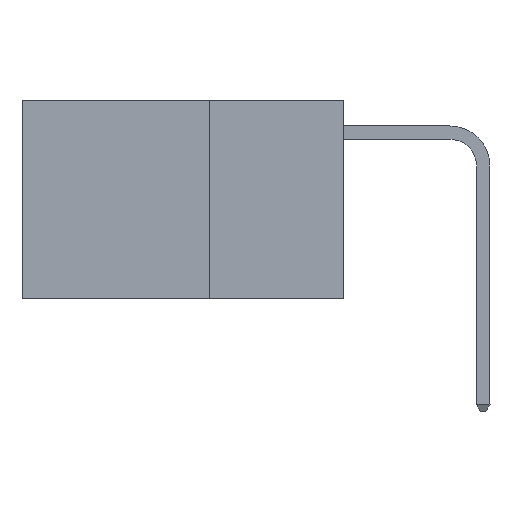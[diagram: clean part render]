
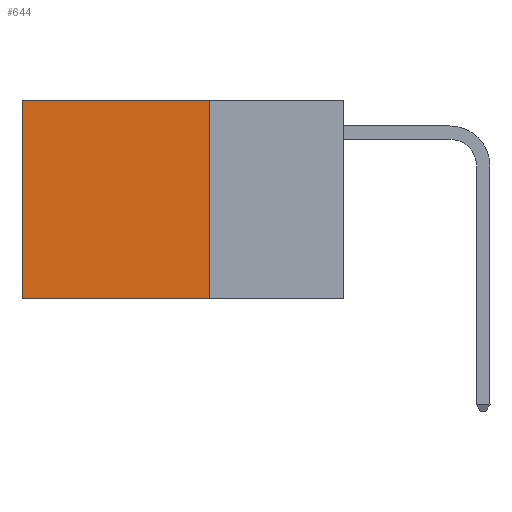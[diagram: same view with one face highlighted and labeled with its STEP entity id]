
A CAD part, left-side view. The second image highlights one B-rep face of the part: STEP entity #644.
In plain terms, the highlighted planar face has unit normal (-1, 0, 0).
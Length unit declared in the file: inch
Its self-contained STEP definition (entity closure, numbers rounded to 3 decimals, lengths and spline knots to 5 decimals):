
#522 = EDGE_CURVE ( 'NONE', #5255, #18764, #23776, .T. ) ;
#644 = ADVANCED_FACE ( 'NONE', ( #17251 ), #6203, .F. ) ;
#690 = VECTOR ( 'NONE', #14482, 39.37008 ) ;
#860 = VECTOR ( 'NONE', #4967, 39.37008 ) ;
#1788 = EDGE_CURVE ( 'NONE', #5255, #20709, #23223, .T. ) ;
#2588 = EDGE_LOOP ( 'NONE', ( #16993, #18044, #10127, #11019 ) ) ;
#2862 = LINE ( 'NONE', #10473, #690 ) ;
#3080 = EDGE_CURVE ( 'NONE', #18764, #13793, #13907, .T. ) ;
#3964 = DIRECTION ( 'NONE',  ( 1., 0., 0. ) ) ;
#4269 = CARTESIAN_POINT ( 'NONE',  ( 0.2625, 0.25, 0. ) ) ;
#4967 = DIRECTION ( 'NONE',  ( 0., 1., 0. ) ) ;
#5255 = VERTEX_POINT ( 'NONE', #6320 ) ;
#6203 = PLANE ( 'NONE',  #22464 ) ;
#6320 = CARTESIAN_POINT ( 'NONE',  ( 0.2625, 0.25, 0. ) ) ;
#6379 = DIRECTION ( 'NONE',  ( 0., 0., -1. ) ) ;
#7777 = VECTOR ( 'NONE', #20364, 39.37008 ) ;
#10127 = ORIENTED_EDGE ( 'NONE', *, *, #1788, .F. ) ;
#10473 = CARTESIAN_POINT ( 'NONE',  ( 0.2625, 0.25, -0.37 ) ) ;
#10672 = CARTESIAN_POINT ( 'NONE',  ( 0.2625, 0.6, -0.37 ) ) ;
#10975 = CARTESIAN_POINT ( 'NONE',  ( 0.2625, 0.6, 0. ) ) ;
#11019 = ORIENTED_EDGE ( 'NONE', *, *, #522, .T. ) ;
#11967 = VECTOR ( 'NONE', #6379, 39.37008 ) ;
#13585 = DIRECTION ( 'NONE',  ( 0., 0., -1. ) ) ;
#13793 = VERTEX_POINT ( 'NONE', #10672 ) ;
#13907 = LINE ( 'NONE', #10975, #7777 ) ;
#14276 = CARTESIAN_POINT ( 'NONE',  ( 0.2625, 0.25, -0.37 ) ) ;
#14482 = DIRECTION ( 'NONE',  ( 0., 1., 0. ) ) ;
#15895 = EDGE_CURVE ( 'NONE', #20709, #13793, #2862, .T. ) ;
#15990 = CARTESIAN_POINT ( 'NONE',  ( 0.2625, 0.25, 0. ) ) ;
#16993 = ORIENTED_EDGE ( 'NONE', *, *, #3080, .T. ) ;
#17126 = CARTESIAN_POINT ( 'NONE',  ( 0.2625, 0.6, 0. ) ) ;
#17251 = FACE_OUTER_BOUND ( 'NONE', #2588, .T. ) ;
#18044 = ORIENTED_EDGE ( 'NONE', *, *, #15895, .F. ) ;
#18764 = VERTEX_POINT ( 'NONE', #17126 ) ;
#20364 = DIRECTION ( 'NONE',  ( 0., 0., -1. ) ) ;
#20709 = VERTEX_POINT ( 'NONE', #14276 ) ;
#22464 = AXIS2_PLACEMENT_3D ( 'NONE', #23039, #3964, #13585 ) ;
#23039 = CARTESIAN_POINT ( 'NONE',  ( 0.2625, 0.25, 0. ) ) ;
#23223 = LINE ( 'NONE', #4269, #11967 ) ;
#23776 = LINE ( 'NONE', #15990, #860 ) ;
